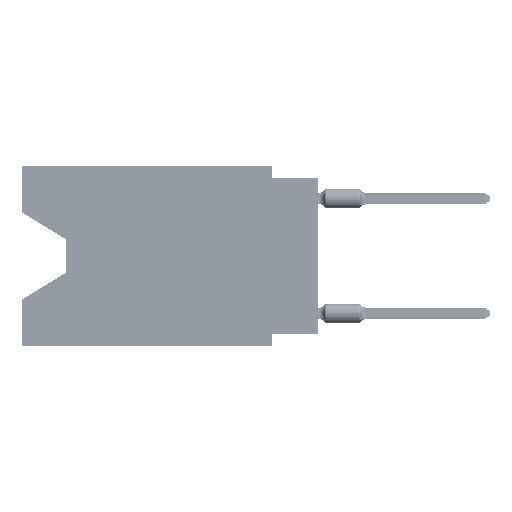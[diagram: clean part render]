
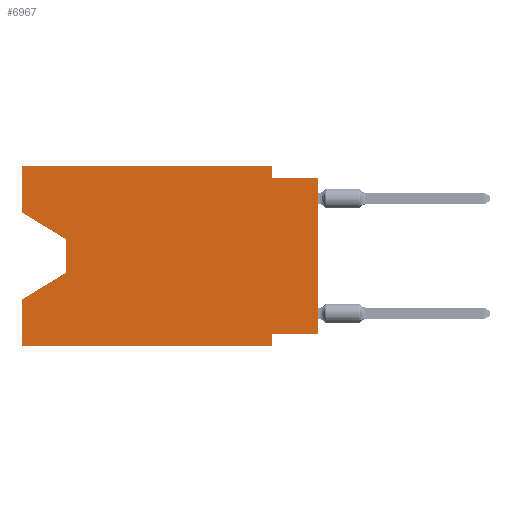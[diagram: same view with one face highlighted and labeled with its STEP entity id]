
A CAD part, left-side view. The second image highlights one B-rep face of the part: STEP entity #6967.
In plain terms, the highlighted planar face has unit normal (-1, 0, 0).
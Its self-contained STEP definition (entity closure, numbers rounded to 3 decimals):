
#1042 = VECTOR ( 'NONE', #51081, 1000. ) ;
#1711 = VECTOR ( 'NONE', #18895, 1000. ) ;
#3283 = CARTESIAN_POINT ( 'NONE',  ( 0., 16.383, -9.906 ) ) ;
#4301 = EDGE_CURVE ( 'NONE', #31980, #69225, #12897, .T. ) ;
#5143 = VERTEX_POINT ( 'NONE', #31322 ) ;
#6967 = ADVANCED_FACE ( 'NONE', ( #7638 ), #32838, .F. ) ;
#7638 = FACE_OUTER_BOUND ( 'NONE', #59796, .T. ) ;
#7884 = ORIENTED_EDGE ( 'NONE', *, *, #34165, .T. ) ;
#8135 = DIRECTION ( 'NONE',  ( 0., 0., -1. ) ) ;
#9288 = CARTESIAN_POINT ( 'NONE',  ( 0., 13.97, -4.013 ) ) ;
#9401 = ORIENTED_EDGE ( 'NONE', *, *, #4301, .T. ) ;
#9477 = VECTOR ( 'NONE', #68193, 1000. ) ;
#10701 = DIRECTION ( 'NONE',  ( 0., -0.855, -0.519 ) ) ;
#11105 = LINE ( 'NONE', #52579, #81137 ) ;
#11515 = EDGE_CURVE ( 'NONE', #69371, #30036, #63481, .T. ) ;
#11685 = DIRECTION ( 'NONE',  ( 0., 0., -1. ) ) ;
#11714 = CARTESIAN_POINT ( 'NONE',  ( 0., 16.383, 0. ) ) ;
#11820 = VERTEX_POINT ( 'NONE', #75788 ) ;
#11821 = ORIENTED_EDGE ( 'NONE', *, *, #11515, .T. ) ;
#12897 = LINE ( 'NONE', #37291, #75642 ) ;
#13289 = EDGE_CURVE ( 'NONE', #31980, #65205, #50692, .T. ) ;
#14067 = LINE ( 'NONE', #11714, #23896 ) ;
#14267 = CARTESIAN_POINT ( 'NONE',  ( 0., 16.383, -7.36 ) ) ;
#17294 = ORIENTED_EDGE ( 'NONE', *, *, #13289, .F. ) ;
#18472 = CARTESIAN_POINT ( 'NONE',  ( 0., 0., 0. ) ) ;
#18647 = VERTEX_POINT ( 'NONE', #73873 ) ;
#18802 = EDGE_CURVE ( 'NONE', #28187, #18647, #63933, .T. ) ;
#18895 = DIRECTION ( 'NONE',  ( 0., 1., 0. ) ) ;
#18953 = VERTEX_POINT ( 'NONE', #36494 ) ;
#19327 = LINE ( 'NONE', #81309, #73911 ) ;
#21823 = CARTESIAN_POINT ( 'NONE',  ( 0., 0., -9.271 ) ) ;
#21864 = EDGE_CURVE ( 'NONE', #42509, #69225, #68292, .T. ) ;
#23608 = CARTESIAN_POINT ( 'NONE',  ( 0., 16.383, 0. ) ) ;
#23650 = EDGE_CURVE ( 'NONE', #69371, #42509, #25108, .T. ) ;
#23896 = VECTOR ( 'NONE', #37327, 1000. ) ;
#24104 = DIRECTION ( 'NONE',  ( 0., -1., 0. ) ) ;
#25108 = LINE ( 'NONE', #62687, #1711 ) ;
#25298 = ORIENTED_EDGE ( 'NONE', *, *, #25964, .T. ) ;
#25964 = EDGE_CURVE ( 'NONE', #45148, #5143, #11105, .T. ) ;
#26376 = VECTOR ( 'NONE', #48762, 1000. ) ;
#28187 = VERTEX_POINT ( 'NONE', #49622 ) ;
#30036 = VERTEX_POINT ( 'NONE', #53970 ) ;
#31322 = CARTESIAN_POINT ( 'NONE',  ( 0., 13.97, -4.013 ) ) ;
#31980 = VERTEX_POINT ( 'NONE', #3283 ) ;
#32838 = PLANE ( 'NONE',  #76002 ) ;
#34165 = EDGE_CURVE ( 'NONE', #11820, #65205, #19327, .T. ) ;
#36140 = ORIENTED_EDGE ( 'NONE', *, *, #18802, .F. ) ;
#36494 = CARTESIAN_POINT ( 'NONE',  ( 0., 16.383, 0. ) ) ;
#37204 = VECTOR ( 'NONE', #79503, 1000. ) ;
#37291 = CARTESIAN_POINT ( 'NONE',  ( 0., 16.383, -9.906 ) ) ;
#37327 = DIRECTION ( 'NONE',  ( 0., 0., 1. ) ) ;
#39841 = EDGE_CURVE ( 'NONE', #45148, #18953, #14067, .T. ) ;
#40892 = EDGE_CURVE ( 'NONE', #5143, #11820, #48084, .T. ) ;
#42509 = VERTEX_POINT ( 'NONE', #54541 ) ;
#42983 = LINE ( 'NONE', #69009, #9477 ) ;
#44421 = ORIENTED_EDGE ( 'NONE', *, *, #23650, .F. ) ;
#45148 = VERTEX_POINT ( 'NONE', #79046 ) ;
#47835 = VECTOR ( 'NONE', #8135, 1000. ) ;
#48084 = LINE ( 'NONE', #9288, #37204 ) ;
#48762 = DIRECTION ( 'NONE',  ( 0., -1., 0. ) ) ;
#49622 = CARTESIAN_POINT ( 'NONE',  ( 0., 2.54, 0. ) ) ;
#50344 = ORIENTED_EDGE ( 'NONE', *, *, #21864, .F. ) ;
#50692 = LINE ( 'NONE', #51499, #51345 ) ;
#51081 = DIRECTION ( 'NONE',  ( 0., 0., 1. ) ) ;
#51345 = VECTOR ( 'NONE', #75911, 1000. ) ;
#51499 = CARTESIAN_POINT ( 'NONE',  ( 0., 16.383, 0. ) ) ;
#51515 = CARTESIAN_POINT ( 'NONE',  ( 0., 2.54, 0. ) ) ;
#52579 = CARTESIAN_POINT ( 'NONE',  ( 0., 16.383, -2.546 ) ) ;
#53065 = DIRECTION ( 'NONE',  ( 1., 0., 0. ) ) ;
#53456 = VECTOR ( 'NONE', #11685, 1000. ) ;
#53970 = CARTESIAN_POINT ( 'NONE',  ( 0., 0., -0.635 ) ) ;
#54541 = CARTESIAN_POINT ( 'NONE',  ( 0., 2.54, -9.271 ) ) ;
#56799 = ORIENTED_EDGE ( 'NONE', *, *, #40892, .T. ) ;
#59198 = EDGE_CURVE ( 'NONE', #18953, #28187, #80178, .T. ) ;
#59796 = EDGE_LOOP ( 'NONE', ( #25298, #56799, #7884, #17294, #9401, #50344, #44421, #11821, #65105, #36140, #65193, #62651 ) ) ;
#61850 = EDGE_CURVE ( 'NONE', #18647, #30036, #42983, .T. ) ;
#62651 = ORIENTED_EDGE ( 'NONE', *, *, #39841, .F. ) ;
#62687 = CARTESIAN_POINT ( 'NONE',  ( 0., 0., -9.271 ) ) ;
#63167 = CARTESIAN_POINT ( 'NONE',  ( 0., 2.54, -9.906 ) ) ;
#63481 = LINE ( 'NONE', #18472, #1042 ) ;
#63933 = LINE ( 'NONE', #51515, #47835 ) ;
#65105 = ORIENTED_EDGE ( 'NONE', *, *, #61850, .F. ) ;
#65193 = ORIENTED_EDGE ( 'NONE', *, *, #59198, .F. ) ;
#65205 = VERTEX_POINT ( 'NONE', #14267 ) ;
#65861 = DIRECTION ( 'NONE',  ( 0., 0., -1. ) ) ;
#68094 = DIRECTION ( 'NONE',  ( 0., 0.855, -0.519 ) ) ;
#68193 = DIRECTION ( 'NONE',  ( 0., -1., 0. ) ) ;
#68292 = LINE ( 'NONE', #74894, #53456 ) ;
#69009 = CARTESIAN_POINT ( 'NONE',  ( 0., 0., -0.635 ) ) ;
#69225 = VERTEX_POINT ( 'NONE', #63167 ) ;
#69371 = VERTEX_POINT ( 'NONE', #21823 ) ;
#73873 = CARTESIAN_POINT ( 'NONE',  ( 0., 2.54, -0.635 ) ) ;
#73911 = VECTOR ( 'NONE', #68094, 1000. ) ;
#74894 = CARTESIAN_POINT ( 'NONE',  ( 0., 2.54, -9.906 ) ) ;
#75642 = VECTOR ( 'NONE', #24104, 1000. ) ;
#75788 = CARTESIAN_POINT ( 'NONE',  ( 0., 13.97, -5.893 ) ) ;
#75911 = DIRECTION ( 'NONE',  ( 0., 0., 1. ) ) ;
#76002 = AXIS2_PLACEMENT_3D ( 'NONE', #79482, #53065, #65861 ) ;
#79046 = CARTESIAN_POINT ( 'NONE',  ( 0., 16.383, -2.546 ) ) ;
#79482 = CARTESIAN_POINT ( 'NONE',  ( 0., 16.383, 0. ) ) ;
#79503 = DIRECTION ( 'NONE',  ( 0., 0., -1. ) ) ;
#80178 = LINE ( 'NONE', #23608, #26376 ) ;
#81137 = VECTOR ( 'NONE', #10701, 1000. ) ;
#81309 = CARTESIAN_POINT ( 'NONE',  ( 0., 13.97, -5.893 ) ) ;
